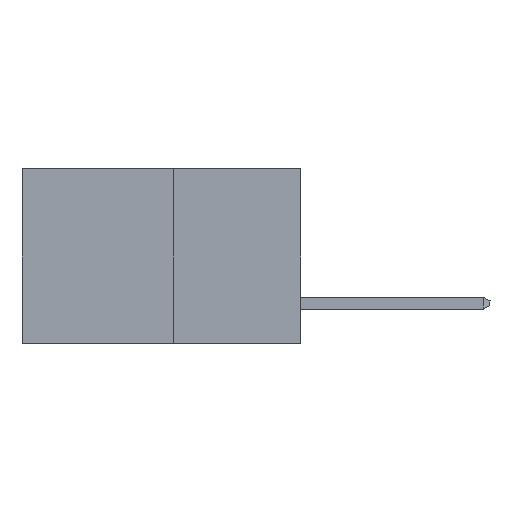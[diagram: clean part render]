
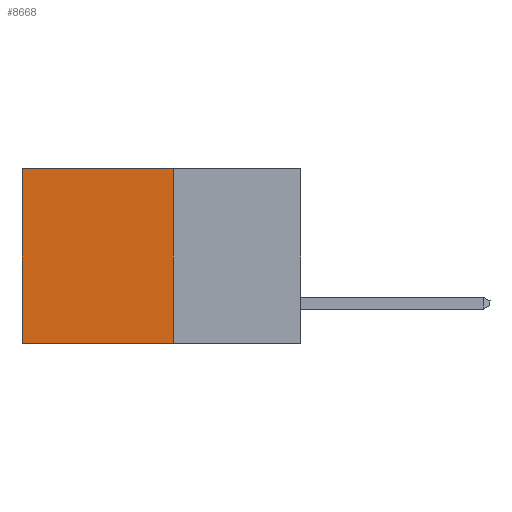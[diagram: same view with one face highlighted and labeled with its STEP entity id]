
A CAD part, left-side view. The second image highlights one B-rep face of the part: STEP entity #8668.
In plain terms, the highlighted planar face has unit normal (-1, 0, 0).
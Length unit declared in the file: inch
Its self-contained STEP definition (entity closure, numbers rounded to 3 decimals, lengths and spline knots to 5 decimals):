
#111 = EDGE_CURVE ( 'NONE', #6174, #3649, #11497, .T. ) ;
#179 = FACE_OUTER_BOUND ( 'NONE', #6884, .T. ) ;
#243 = CARTESIAN_POINT ( 'NONE',  ( 0.277, 0.27, 0. ) ) ;
#305 = VECTOR ( 'NONE', #6578, 39.37008 ) ;
#461 = VERTEX_POINT ( 'NONE', #243 ) ;
#1059 = CARTESIAN_POINT ( 'NONE',  ( 0.277, 0.27, -0.37 ) ) ;
#1420 = ORIENTED_EDGE ( 'NONE', *, *, #111, .T. ) ;
#1818 = EDGE_CURVE ( 'NONE', #461, #6174, #3177, .T. ) ;
#2285 = EDGE_CURVE ( 'NONE', #461, #4382, #12200, .T. ) ;
#2374 = VECTOR ( 'NONE', #12488, 39.37008 ) ;
#3177 = LINE ( 'NONE', #8134, #305 ) ;
#3649 = VERTEX_POINT ( 'NONE', #5858 ) ;
#4147 = EDGE_CURVE ( 'NONE', #4382, #3649, #10208, .T. ) ;
#4382 = VERTEX_POINT ( 'NONE', #9899 ) ;
#4550 = ORIENTED_EDGE ( 'NONE', *, *, #2285, .F. ) ;
#5858 = CARTESIAN_POINT ( 'NONE',  ( 0.277, 0.59, -0.37 ) ) ;
#6174 = VERTEX_POINT ( 'NONE', #10182 ) ;
#6560 = VECTOR ( 'NONE', #11141, 39.37008 ) ;
#6578 = DIRECTION ( 'NONE',  ( 0., 1., 0. ) ) ;
#6884 = EDGE_LOOP ( 'NONE', ( #1420, #8830, #4550, #10721 ) ) ;
#7193 = CARTESIAN_POINT ( 'NONE',  ( 0.277, 0.59, -0.37 ) ) ;
#7438 = CARTESIAN_POINT ( 'NONE',  ( 0.277, 0.27, -0.37 ) ) ;
#7944 = DIRECTION ( 'NONE',  ( 1., 0., 0. ) ) ;
#8134 = CARTESIAN_POINT ( 'NONE',  ( 0.277, 0.27, 0. ) ) ;
#8668 = ADVANCED_FACE ( 'NONE', ( #179 ), #8906, .F. ) ;
#8830 = ORIENTED_EDGE ( 'NONE', *, *, #4147, .F. ) ;
#8906 = PLANE ( 'NONE',  #11713 ) ;
#9781 = CARTESIAN_POINT ( 'NONE',  ( 0.277, 0.27, -0.37 ) ) ;
#9896 = VECTOR ( 'NONE', #12100, 39.37008 ) ;
#9899 = CARTESIAN_POINT ( 'NONE',  ( 0.277, 0.27, -0.37 ) ) ;
#10182 = CARTESIAN_POINT ( 'NONE',  ( 0.277, 0.59, 0. ) ) ;
#10208 = LINE ( 'NONE', #1059, #9896 ) ;
#10721 = ORIENTED_EDGE ( 'NONE', *, *, #1818, .T. ) ;
#11141 = DIRECTION ( 'NONE',  ( 0., 0., -1. ) ) ;
#11497 = LINE ( 'NONE', #7193, #6560 ) ;
#11713 = AXIS2_PLACEMENT_3D ( 'NONE', #9781, #7944, #12375 ) ;
#12100 = DIRECTION ( 'NONE',  ( 0., 1., 0. ) ) ;
#12200 = LINE ( 'NONE', #7438, #2374 ) ;
#12375 = DIRECTION ( 'NONE',  ( 0., 0., -1. ) ) ;
#12488 = DIRECTION ( 'NONE',  ( 0., 0., -1. ) ) ;
